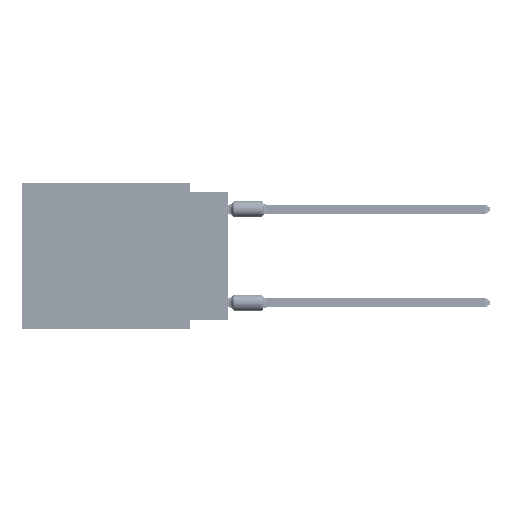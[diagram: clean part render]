
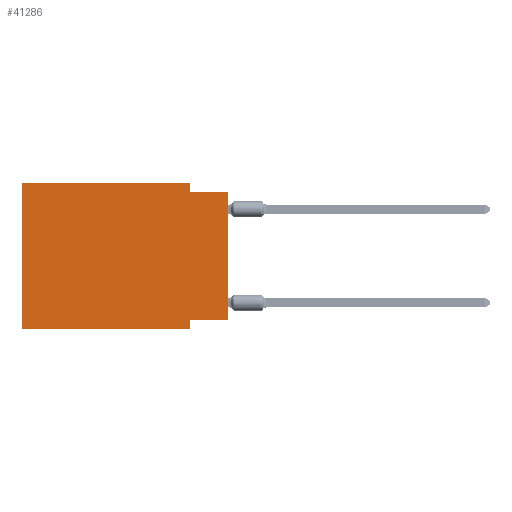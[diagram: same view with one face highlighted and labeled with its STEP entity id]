
A CAD part, left-side view. The second image highlights one B-rep face of the part: STEP entity #41286.
In plain terms, the highlighted planar face has unit normal (-1, 0, 0).
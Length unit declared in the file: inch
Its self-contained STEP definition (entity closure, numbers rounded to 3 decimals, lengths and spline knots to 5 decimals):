
#1385 = CARTESIAN_POINT ( 'NONE',  ( 0., 0.1, -0.025 ) ) ;
#2822 = CARTESIAN_POINT ( 'NONE',  ( 0., 0.1, -0.365 ) ) ;
#4592 = EDGE_CURVE ( 'NONE', #45229, #65723, #43168, .T. ) ;
#5917 = CARTESIAN_POINT ( 'NONE',  ( 0., 0.55, 0. ) ) ;
#10880 = FACE_OUTER_BOUND ( 'NONE', #51571, .T. ) ;
#11273 = LINE ( 'NONE', #5917, #18103 ) ;
#11571 = ORIENTED_EDGE ( 'NONE', *, *, #59110, .F. ) ;
#11785 = EDGE_CURVE ( 'NONE', #53525, #52665, #11273, .T. ) ;
#13224 = CARTESIAN_POINT ( 'NONE',  ( 0., 0.1, -0.39 ) ) ;
#13487 = LINE ( 'NONE', #46631, #63189 ) ;
#13614 = DIRECTION ( 'NONE',  ( 0., 0., -1. ) ) ;
#14530 = DIRECTION ( 'NONE',  ( 0., 0., 1. ) ) ;
#15376 = ORIENTED_EDGE ( 'NONE', *, *, #11785, .F. ) ;
#15850 = CARTESIAN_POINT ( 'NONE',  ( 0., 0.55, -0.39 ) ) ;
#16839 = CARTESIAN_POINT ( 'NONE',  ( 0., 0.55, 0. ) ) ;
#17097 = CARTESIAN_POINT ( 'NONE',  ( 0., 0.1, 0. ) ) ;
#18103 = VECTOR ( 'NONE', #34040, 39.37008 ) ;
#18543 = VERTEX_POINT ( 'NONE', #15850 ) ;
#19618 = EDGE_CURVE ( 'NONE', #18543, #53525, #13487, .T. ) ;
#20064 = LINE ( 'NONE', #30023, #36148 ) ;
#23191 = EDGE_CURVE ( 'NONE', #45229, #50522, #62518, .T. ) ;
#24287 = LINE ( 'NONE', #62451, #59464 ) ;
#27190 = EDGE_CURVE ( 'NONE', #18543, #56756, #59368, .T. ) ;
#27272 = PLANE ( 'NONE',  #66990 ) ;
#28707 = ORIENTED_EDGE ( 'NONE', *, *, #40264, .F. ) ;
#29288 = VERTEX_POINT ( 'NONE', #1385 ) ;
#30023 = CARTESIAN_POINT ( 'NONE',  ( 0., 0., -0.025 ) ) ;
#31344 = VECTOR ( 'NONE', #61841, 39.37008 ) ;
#33873 = CARTESIAN_POINT ( 'NONE',  ( 0., 0., 0. ) ) ;
#34040 = DIRECTION ( 'NONE',  ( 0., -1., 0. ) ) ;
#34644 = VECTOR ( 'NONE', #35399, 39.37008 ) ;
#34869 = CARTESIAN_POINT ( 'NONE',  ( 0., 0., -0.025 ) ) ;
#35399 = DIRECTION ( 'NONE',  ( 0., 1., 0. ) ) ;
#36148 = VECTOR ( 'NONE', #68552, 39.37008 ) ;
#36474 = VECTOR ( 'NONE', #65609, 39.37008 ) ;
#37247 = DIRECTION ( 'NONE',  ( 1., 0., 0. ) ) ;
#37391 = EDGE_CURVE ( 'NONE', #50522, #56756, #50439, .T. ) ;
#39690 = CARTESIAN_POINT ( 'NONE',  ( 0., 0.55, -0.39 ) ) ;
#40071 = CARTESIAN_POINT ( 'NONE',  ( 0., 0.1, -0.39 ) ) ;
#40264 = EDGE_CURVE ( 'NONE', #29288, #65723, #20064, .T. ) ;
#41286 = ADVANCED_FACE ( 'NONE', ( #10880 ), #27272, .F. ) ;
#43168 = LINE ( 'NONE', #33873, #36474 ) ;
#43984 = DIRECTION ( 'NONE',  ( 0., -1., 0. ) ) ;
#45229 = VERTEX_POINT ( 'NONE', #60778 ) ;
#46631 = CARTESIAN_POINT ( 'NONE',  ( 0., 0.55, 0. ) ) ;
#50439 = LINE ( 'NONE', #40071, #31344 ) ;
#50522 = VERTEX_POINT ( 'NONE', #2822 ) ;
#51571 = EDGE_LOOP ( 'NONE', ( #57041, #28707, #11571, #15376, #65333, #66825, #63583, #56389 ) ) ;
#52665 = VERTEX_POINT ( 'NONE', #17097 ) ;
#53525 = VERTEX_POINT ( 'NONE', #16839 ) ;
#56389 = ORIENTED_EDGE ( 'NONE', *, *, #23191, .F. ) ;
#56482 = VECTOR ( 'NONE', #43984, 39.37008 ) ;
#56756 = VERTEX_POINT ( 'NONE', #13224 ) ;
#57041 = ORIENTED_EDGE ( 'NONE', *, *, #4592, .T. ) ;
#59110 = EDGE_CURVE ( 'NONE', #52665, #29288, #24287, .T. ) ;
#59368 = LINE ( 'NONE', #39690, #56482 ) ;
#59464 = VECTOR ( 'NONE', #13614, 39.37008 ) ;
#60778 = CARTESIAN_POINT ( 'NONE',  ( 0., 0., -0.365 ) ) ;
#61841 = DIRECTION ( 'NONE',  ( 0., 0., -1. ) ) ;
#62153 = CARTESIAN_POINT ( 'NONE',  ( 0., 0., -0.365 ) ) ;
#62451 = CARTESIAN_POINT ( 'NONE',  ( 0., 0.1, 0. ) ) ;
#62518 = LINE ( 'NONE', #62153, #34644 ) ;
#63189 = VECTOR ( 'NONE', #14530, 39.37008 ) ;
#63583 = ORIENTED_EDGE ( 'NONE', *, *, #37391, .F. ) ;
#65333 = ORIENTED_EDGE ( 'NONE', *, *, #19618, .F. ) ;
#65609 = DIRECTION ( 'NONE',  ( 0., 0., 1. ) ) ;
#65723 = VERTEX_POINT ( 'NONE', #34869 ) ;
#66118 = CARTESIAN_POINT ( 'NONE',  ( 0., 0.55, 0. ) ) ;
#66455 = DIRECTION ( 'NONE',  ( 0., 0., -1. ) ) ;
#66825 = ORIENTED_EDGE ( 'NONE', *, *, #27190, .T. ) ;
#66990 = AXIS2_PLACEMENT_3D ( 'NONE', #66118, #37247, #66455 ) ;
#68552 = DIRECTION ( 'NONE',  ( 0., -1., 0. ) ) ;
